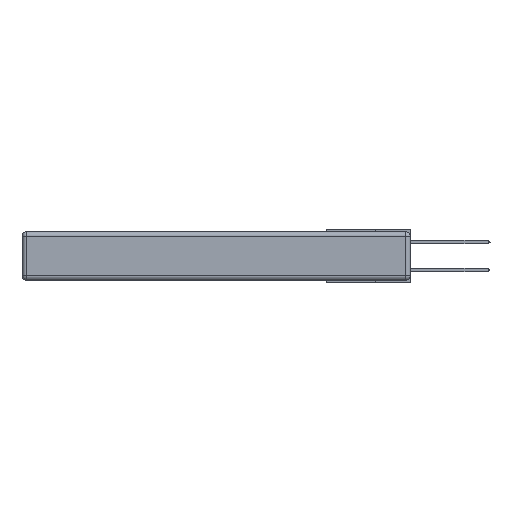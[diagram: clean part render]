
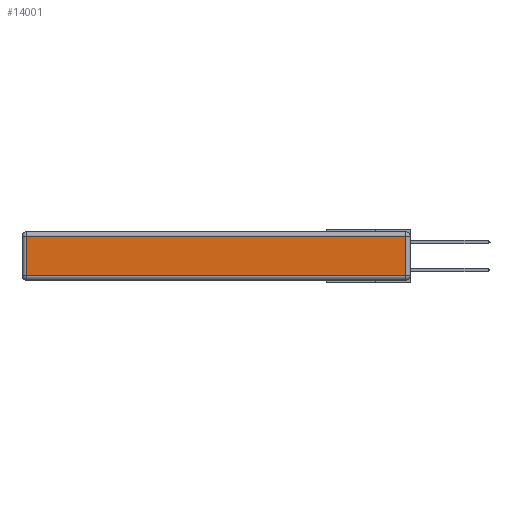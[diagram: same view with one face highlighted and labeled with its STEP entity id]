
A CAD part, left-side view. The second image highlights one B-rep face of the part: STEP entity #14001.
In plain terms, the highlighted planar face has unit normal (-1, 0, 0).
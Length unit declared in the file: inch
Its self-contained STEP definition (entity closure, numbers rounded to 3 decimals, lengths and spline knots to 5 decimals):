
#70 = CARTESIAN_POINT ( 'NONE',  ( 0., 2.72, -0.03 ) ) ;
#77 = CARTESIAN_POINT ( 'NONE',  ( 0., 0.03, -0.313 ) ) ;
#959 = LINE ( 'NONE', #9996, #12769 ) ;
#2369 = ORIENTED_EDGE ( 'NONE', *, *, #2536, .T. ) ;
#2470 = CARTESIAN_POINT ( 'NONE',  ( 0., 2.72, -0.313 ) ) ;
#2536 = EDGE_CURVE ( 'NONE', #14087, #12747, #12048, .T. ) ;
#3071 = ORIENTED_EDGE ( 'NONE', *, *, #10625, .T. ) ;
#3199 = EDGE_LOOP ( 'NONE', ( #17908, #2369, #15016, #3071 ) ) ;
#3370 = EDGE_CURVE ( 'NONE', #12747, #4924, #17637, .T. ) ;
#3604 = CARTESIAN_POINT ( 'NONE',  ( 0., 0.03, -0.03 ) ) ;
#3895 = AXIS2_PLACEMENT_3D ( 'NONE', #8939, #9142, #9260 ) ;
#3911 = FACE_OUTER_BOUND ( 'NONE', #3199, .T. ) ;
#4924 = VERTEX_POINT ( 'NONE', #70 ) ;
#6739 = CARTESIAN_POINT ( 'NONE',  ( 0., 0.03, -0.343 ) ) ;
#8691 = LINE ( 'NONE', #19593, #17580 ) ;
#8939 = CARTESIAN_POINT ( 'NONE',  ( 0., 0., -0.343 ) ) ;
#9007 = PLANE ( 'NONE',  #3895 ) ;
#9142 = DIRECTION ( 'NONE',  ( -1., 0., 0. ) ) ;
#9260 = DIRECTION ( 'NONE',  ( 0., 0., 1. ) ) ;
#9996 = CARTESIAN_POINT ( 'NONE',  ( 0., 2.72, -0.343 ) ) ;
#10586 = VECTOR ( 'NONE', #17444, 39.37008 ) ;
#10625 = EDGE_CURVE ( 'NONE', #4924, #16535, #959, .T. ) ;
#11777 = DIRECTION ( 'NONE',  ( 0., 1., 0. ) ) ;
#12048 = LINE ( 'NONE', #6739, #10586 ) ;
#12747 = VERTEX_POINT ( 'NONE', #3604 ) ;
#12769 = VECTOR ( 'NONE', #14635, 39.37008 ) ;
#14001 = ADVANCED_FACE ( 'NONE', ( #3911 ), #9007, .T. ) ;
#14087 = VERTEX_POINT ( 'NONE', #77 ) ;
#14635 = DIRECTION ( 'NONE',  ( 0., 0., -1. ) ) ;
#15016 = ORIENTED_EDGE ( 'NONE', *, *, #3370, .T. ) ;
#15185 = DIRECTION ( 'NONE',  ( 0., -1., 0. ) ) ;
#16434 = VECTOR ( 'NONE', #11777, 39.37008 ) ;
#16535 = VERTEX_POINT ( 'NONE', #2470 ) ;
#17444 = DIRECTION ( 'NONE',  ( 0., 0., 1. ) ) ;
#17580 = VECTOR ( 'NONE', #15185, 39.37008 ) ;
#17637 = LINE ( 'NONE', #19452, #16434 ) ;
#17908 = ORIENTED_EDGE ( 'NONE', *, *, #18066, .T. ) ;
#18066 = EDGE_CURVE ( 'NONE', #16535, #14087, #8691, .T. ) ;
#19452 = CARTESIAN_POINT ( 'NONE',  ( 0., 2.75, -0.03 ) ) ;
#19593 = CARTESIAN_POINT ( 'NONE',  ( 0., 0., -0.313 ) ) ;
